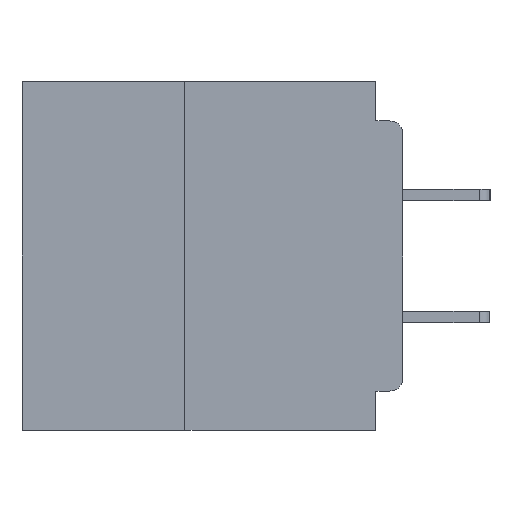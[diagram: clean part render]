
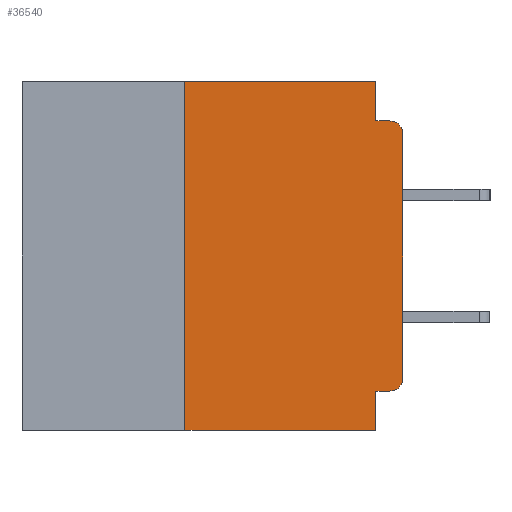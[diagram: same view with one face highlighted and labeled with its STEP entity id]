
A CAD part, left-side view. The second image highlights one B-rep face of the part: STEP entity #36540.
In plain terms, the highlighted planar face has unit normal (-1, 0, 0).
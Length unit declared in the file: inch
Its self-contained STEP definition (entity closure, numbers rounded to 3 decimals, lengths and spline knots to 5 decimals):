
#18 = LINE ( 'NONE', #40953, #2610 ) ;
#345 = VERTEX_POINT ( 'NONE', #15769 ) ;
#551 = EDGE_CURVE ( 'NONE', #43628, #2626, #37758, .T. ) ;
#800 = DIRECTION ( 'NONE',  ( 0., 1., 0. ) ) ;
#1693 = AXIS2_PLACEMENT_3D ( 'NONE', #5947, #34654, #10143 ) ;
#2564 = CARTESIAN_POINT ( 'NONE',  ( 0., 0., -0.34 ) ) ;
#2610 = VECTOR ( 'NONE', #16509, 39.37008 ) ;
#2626 = VERTEX_POINT ( 'NONE', #47192 ) ;
#3548 = VERTEX_POINT ( 'NONE', #2564 ) ;
#4885 = LINE ( 'NONE', #30077, #47214 ) ;
#5537 = CARTESIAN_POINT ( 'NONE',  ( 0., 0.031, -0.045 ) ) ;
#5947 = CARTESIAN_POINT ( 'NONE',  ( 0., 0.015, -0.34 ) ) ;
#6094 = EDGE_CURVE ( 'NONE', #43049, #47334, #23448, .T. ) ;
#6746 = VECTOR ( 'NONE', #18537, 39.37008 ) ;
#6789 = LINE ( 'NONE', #19108, #49099 ) ;
#7345 = DIRECTION ( 'NONE',  ( 0., 0., -1. ) ) ;
#7756 = ORIENTED_EDGE ( 'NONE', *, *, #31860, .T. ) ;
#8455 = ORIENTED_EDGE ( 'NONE', *, *, #38276, .F. ) ;
#9150 = ORIENTED_EDGE ( 'NONE', *, *, #38666, .F. ) ;
#10143 = DIRECTION ( 'NONE',  ( 0., 0., -1. ) ) ;
#11046 = VECTOR ( 'NONE', #29273, 39.37008 ) ;
#11926 = EDGE_CURVE ( 'NONE', #15871, #47334, #40742, .T. ) ;
#14401 = CARTESIAN_POINT ( 'NONE',  ( 0., 0.031, -0.4 ) ) ;
#14569 = ORIENTED_EDGE ( 'NONE', *, *, #40596, .T. ) ;
#14743 = ORIENTED_EDGE ( 'NONE', *, *, #20010, .T. ) ;
#15769 = CARTESIAN_POINT ( 'NONE',  ( 0., 0.25, 0. ) ) ;
#15871 = VERTEX_POINT ( 'NONE', #42211 ) ;
#16509 = DIRECTION ( 'NONE',  ( 0., 0., 1. ) ) ;
#17922 = DIRECTION ( 'NONE',  ( 0., 0., -1. ) ) ;
#18537 = DIRECTION ( 'NONE',  ( 0., 0., -1. ) ) ;
#18975 = VECTOR ( 'NONE', #29792, 39.37008 ) ;
#19108 = CARTESIAN_POINT ( 'NONE',  ( 0., 0.437, -0.4 ) ) ;
#19200 = EDGE_LOOP ( 'NONE', ( #14743, #38145, #23160, #36739, #9150, #34996, #7756, #8455, #36356, #14569 ) ) ;
#19407 = CARTESIAN_POINT ( 'NONE',  ( 0., 0.015, -0.06 ) ) ;
#19733 = DIRECTION ( 'NONE',  ( 0., -1., 0. ) ) ;
#20010 = EDGE_CURVE ( 'NONE', #3548, #15871, #18, .T. ) ;
#20502 = FACE_OUTER_BOUND ( 'NONE', #19200, .T. ) ;
#20693 = CIRCLE ( 'NONE', #1693, 0.015 ) ;
#23160 = ORIENTED_EDGE ( 'NONE', *, *, #6094, .F. ) ;
#23229 = CARTESIAN_POINT ( 'NONE',  ( 0., 0.015, -0.045 ) ) ;
#23426 = AXIS2_PLACEMENT_3D ( 'NONE', #19407, #47983, #23526 ) ;
#23448 = LINE ( 'NONE', #40190, #43858 ) ;
#23526 = DIRECTION ( 'NONE',  ( 0., 0., -1. ) ) ;
#23750 = PLANE ( 'NONE',  #34343 ) ;
#23791 = VERTEX_POINT ( 'NONE', #27277 ) ;
#25677 = CARTESIAN_POINT ( 'NONE',  ( 0., 0.437, 0. ) ) ;
#27114 = CARTESIAN_POINT ( 'NONE',  ( 0., 0.015, -0.355 ) ) ;
#27277 = CARTESIAN_POINT ( 'NONE',  ( 0., 0.031, -0.4 ) ) ;
#28645 = LINE ( 'NONE', #14401, #6746 ) ;
#29273 = DIRECTION ( 'NONE',  ( 0., 0., 1. ) ) ;
#29792 = DIRECTION ( 'NONE',  ( 0., -1., 0. ) ) ;
#30077 = CARTESIAN_POINT ( 'NONE',  ( 0., 0.031, 0. ) ) ;
#31860 = EDGE_CURVE ( 'NONE', #46163, #23791, #6789, .T. ) ;
#31948 = DIRECTION ( 'NONE',  ( 1., 0., 0. ) ) ;
#33015 = CARTESIAN_POINT ( 'NONE',  ( 0., 0.031, 0. ) ) ;
#33366 = CARTESIAN_POINT ( 'NONE',  ( 0., 0.25, -0.4 ) ) ;
#34343 = AXIS2_PLACEMENT_3D ( 'NONE', #39965, #31948, #7345 ) ;
#34654 = DIRECTION ( 'NONE',  ( -1., 0., 0. ) ) ;
#34827 = EDGE_CURVE ( 'NONE', #46163, #345, #43673, .T. ) ;
#34996 = ORIENTED_EDGE ( 'NONE', *, *, #34827, .F. ) ;
#35782 = CARTESIAN_POINT ( 'NONE',  ( 0., 0.25, -0.4 ) ) ;
#36356 = ORIENTED_EDGE ( 'NONE', *, *, #551, .F. ) ;
#36475 = VECTOR ( 'NONE', #800, 39.37008 ) ;
#36540 = ADVANCED_FACE ( 'NONE', ( #20502 ), #23750, .F. ) ;
#36739 = ORIENTED_EDGE ( 'NONE', *, *, #46003, .F. ) ;
#37747 = CARTESIAN_POINT ( 'NONE',  ( 0., 0., -0.355 ) ) ;
#37758 = LINE ( 'NONE', #37747, #36475 ) ;
#38145 = ORIENTED_EDGE ( 'NONE', *, *, #11926, .T. ) ;
#38276 = EDGE_CURVE ( 'NONE', #2626, #23791, #28645, .T. ) ;
#38666 = EDGE_CURVE ( 'NONE', #345, #41009, #51553, .T. ) ;
#39965 = CARTESIAN_POINT ( 'NONE',  ( 0., 0.437, 0. ) ) ;
#40190 = CARTESIAN_POINT ( 'NONE',  ( 0., 0., -0.045 ) ) ;
#40596 = EDGE_CURVE ( 'NONE', #43628, #3548, #20693, .T. ) ;
#40742 = CIRCLE ( 'NONE', #23426, 0.015 ) ;
#40953 = CARTESIAN_POINT ( 'NONE',  ( 0., 0., 0. ) ) ;
#41009 = VERTEX_POINT ( 'NONE', #33015 ) ;
#42211 = CARTESIAN_POINT ( 'NONE',  ( 0., 0., -0.06 ) ) ;
#43049 = VERTEX_POINT ( 'NONE', #5537 ) ;
#43628 = VERTEX_POINT ( 'NONE', #27114 ) ;
#43673 = LINE ( 'NONE', #33366, #11046 ) ;
#43858 = VECTOR ( 'NONE', #48426, 39.37008 ) ;
#46003 = EDGE_CURVE ( 'NONE', #41009, #43049, #4885, .T. ) ;
#46163 = VERTEX_POINT ( 'NONE', #35782 ) ;
#47192 = CARTESIAN_POINT ( 'NONE',  ( 0., 0.031, -0.355 ) ) ;
#47214 = VECTOR ( 'NONE', #17922, 39.37008 ) ;
#47334 = VERTEX_POINT ( 'NONE', #23229 ) ;
#47983 = DIRECTION ( 'NONE',  ( -1., 0., 0. ) ) ;
#48426 = DIRECTION ( 'NONE',  ( 0., -1., 0. ) ) ;
#49099 = VECTOR ( 'NONE', #19733, 39.37008 ) ;
#51553 = LINE ( 'NONE', #25677, #18975 ) ;
